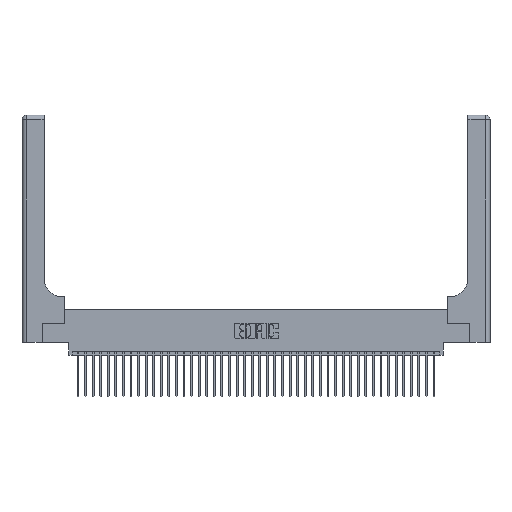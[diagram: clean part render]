
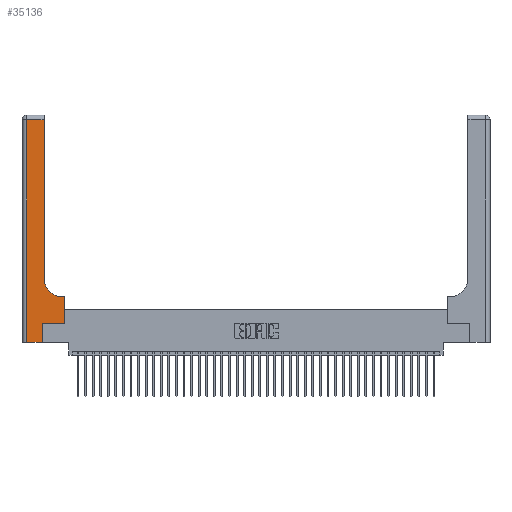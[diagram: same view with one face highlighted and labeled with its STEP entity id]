
A CAD part, top view. The second image highlights one B-rep face of the part: STEP entity #35136.
In plain terms, the highlighted planar face has unit normal (0, 0, 1).
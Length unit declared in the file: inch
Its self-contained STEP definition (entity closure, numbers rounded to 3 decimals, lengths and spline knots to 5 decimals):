
#342 = LINE ( 'NONE', #4594, #36511 ) ;
#909 = LINE ( 'NONE', #28514, #35601 ) ;
#1025 = ORIENTED_EDGE ( 'NONE', *, *, #38267, .T. ) ;
#1485 = CARTESIAN_POINT ( 'NONE',  ( 0.2915, 3., 0.37 ) ) ;
#1682 = DIRECTION ( 'NONE',  ( 0., 0., -1. ) ) ;
#1941 = CARTESIAN_POINT ( 'NONE',  ( 0., 3., 0.37 ) ) ;
#2284 = VECTOR ( 'NONE', #30977, 39.37008 ) ;
#2611 = DIRECTION ( 'NONE',  ( 0., 1., 0. ) ) ;
#2664 = AXIS2_PLACEMENT_3D ( 'NONE', #1941, #1682, #34600 ) ;
#2738 = CARTESIAN_POINT ( 'NONE',  ( 0.5415, 0.6, 0.37 ) ) ;
#3147 = VERTEX_POINT ( 'NONE', #2738 ) ;
#4594 = CARTESIAN_POINT ( 'NONE',  ( 0., 0., 0.37 ) ) ;
#6976 = VECTOR ( 'NONE', #27553, 39.37008 ) ;
#7623 = EDGE_CURVE ( 'NONE', #39054, #41125, #342, .T. ) ;
#8216 = CARTESIAN_POINT ( 'NONE',  ( 0.2915, 2.94, 0.37 ) ) ;
#8793 = ORIENTED_EDGE ( 'NONE', *, *, #41791, .T. ) ;
#9041 = VECTOR ( 'NONE', #22657, 39.37008 ) ;
#9489 = CARTESIAN_POINT ( 'NONE',  ( 0.06, 0., 0.37 ) ) ;
#10050 = ORIENTED_EDGE ( 'NONE', *, *, #30638, .T. ) ;
#10993 = VERTEX_POINT ( 'NONE', #26802 ) ;
#12130 = CARTESIAN_POINT ( 'NONE',  ( 0.06, 2.94, 0.37 ) ) ;
#12388 = CARTESIAN_POINT ( 'NONE',  ( 0.269, 0.25, 0.37 ) ) ;
#12641 = CARTESIAN_POINT ( 'NONE',  ( 0.06, 3., 0.37 ) ) ;
#13434 = VERTEX_POINT ( 'NONE', #37950 ) ;
#14338 = VECTOR ( 'NONE', #2611, 39.37008 ) ;
#14599 = PLANE ( 'NONE',  #2664 ) ;
#14909 = LINE ( 'NONE', #12388, #27704 ) ;
#15469 = VERTEX_POINT ( 'NONE', #12130 ) ;
#16427 = CARTESIAN_POINT ( 'NONE',  ( 0.5585, 0.6, 0.37 ) ) ;
#17239 = DIRECTION ( 'NONE',  ( 1., 0., 0. ) ) ;
#17317 = CIRCLE ( 'NONE', #27830, 0.25 ) ;
#19159 = CARTESIAN_POINT ( 'NONE',  ( 0.2915, 0.85, 0.37 ) ) ;
#19203 = DIRECTION ( 'NONE',  ( -1., 0., 0. ) ) ;
#19743 = VERTEX_POINT ( 'NONE', #19159 ) ;
#20312 = VERTEX_POINT ( 'NONE', #8216 ) ;
#20354 = EDGE_LOOP ( 'NONE', ( #27481, #28086, #41819, #30532, #29692, #1025, #10050, #8793, #29550 ) ) ;
#21682 = DIRECTION ( 'NONE',  ( 1., 0., 0. ) ) ;
#22124 = CARTESIAN_POINT ( 'NONE',  ( 0.5585, 0.25, 0.37 ) ) ;
#22657 = DIRECTION ( 'NONE',  ( 0., -1., 0. ) ) ;
#24025 = CARTESIAN_POINT ( 'NONE',  ( 0.5415, 0.85, 0.37 ) ) ;
#24878 = LINE ( 'NONE', #1485, #6976 ) ;
#24896 = EDGE_CURVE ( 'NONE', #3147, #19743, #17317, .T. ) ;
#25400 = LINE ( 'NONE', #12641, #9041 ) ;
#26802 = CARTESIAN_POINT ( 'NONE',  ( 0.5585, 0.25, 0.37 ) ) ;
#27331 = EDGE_CURVE ( 'NONE', #19743, #20312, #24878, .T. ) ;
#27481 = ORIENTED_EDGE ( 'NONE', *, *, #27331, .T. ) ;
#27553 = DIRECTION ( 'NONE',  ( 0., 1., 0. ) ) ;
#27654 = CARTESIAN_POINT ( 'NONE',  ( 0., 2.94, 0.37 ) ) ;
#27702 = LINE ( 'NONE', #27876, #28714 ) ;
#27704 = VECTOR ( 'NONE', #21682, 39.37008 ) ;
#27744 = DIRECTION ( 'NONE',  ( 0., 1., 0. ) ) ;
#27830 = AXIS2_PLACEMENT_3D ( 'NONE', #24025, #30346, #28163 ) ;
#27876 = CARTESIAN_POINT ( 'NONE',  ( 0.269, 0., 0.37 ) ) ;
#28086 = ORIENTED_EDGE ( 'NONE', *, *, #29153, .T. ) ;
#28163 = DIRECTION ( 'NONE',  ( 1., 0., 0. ) ) ;
#28514 = CARTESIAN_POINT ( 'NONE',  ( 0.2915, 0.6, 0.37 ) ) ;
#28714 = VECTOR ( 'NONE', #27744, 39.37008 ) ;
#29153 = EDGE_CURVE ( 'NONE', #20312, #15469, #38995, .T. ) ;
#29550 = ORIENTED_EDGE ( 'NONE', *, *, #24896, .T. ) ;
#29692 = ORIENTED_EDGE ( 'NONE', *, *, #39383, .T. ) ;
#30070 = VERTEX_POINT ( 'NONE', #16427 ) ;
#30346 = DIRECTION ( 'NONE',  ( 0., 0., -1. ) ) ;
#30532 = ORIENTED_EDGE ( 'NONE', *, *, #7623, .T. ) ;
#30638 = EDGE_CURVE ( 'NONE', #10993, #30070, #40413, .T. ) ;
#30977 = DIRECTION ( 'NONE',  ( -1., 0., 0. ) ) ;
#31542 = FACE_OUTER_BOUND ( 'NONE', #20354, .T. ) ;
#34600 = DIRECTION ( 'NONE',  ( -1., 0., 0. ) ) ;
#35136 = ADVANCED_FACE ( 'NONE', ( #31542 ), #14599, .F. ) ;
#35601 = VECTOR ( 'NONE', #19203, 39.37008 ) ;
#36318 = CARTESIAN_POINT ( 'NONE',  ( 0.269, 0., 0.37 ) ) ;
#36511 = VECTOR ( 'NONE', #17239, 39.37008 ) ;
#37950 = CARTESIAN_POINT ( 'NONE',  ( 0.269, 0.25, 0.37 ) ) ;
#38267 = EDGE_CURVE ( 'NONE', #13434, #10993, #14909, .T. ) ;
#38995 = LINE ( 'NONE', #27654, #2284 ) ;
#39054 = VERTEX_POINT ( 'NONE', #9489 ) ;
#39383 = EDGE_CURVE ( 'NONE', #41125, #13434, #27702, .T. ) ;
#40413 = LINE ( 'NONE', #22124, #14338 ) ;
#41125 = VERTEX_POINT ( 'NONE', #36318 ) ;
#41791 = EDGE_CURVE ( 'NONE', #30070, #3147, #909, .T. ) ;
#41819 = ORIENTED_EDGE ( 'NONE', *, *, #41838, .T. ) ;
#41838 = EDGE_CURVE ( 'NONE', #15469, #39054, #25400, .T. ) ;
